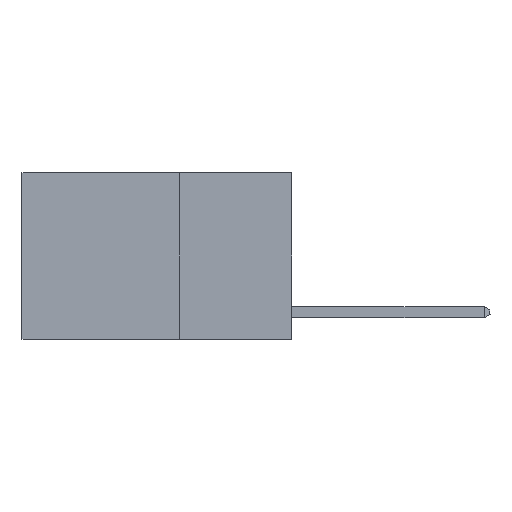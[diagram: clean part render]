
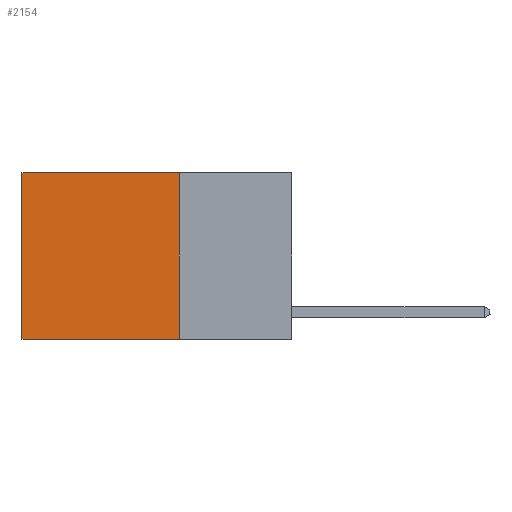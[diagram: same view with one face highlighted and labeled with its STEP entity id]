
A CAD part, left-side view. The second image highlights one B-rep face of the part: STEP entity #2154.
In plain terms, the highlighted planar face has unit normal (-1, 0, 0).
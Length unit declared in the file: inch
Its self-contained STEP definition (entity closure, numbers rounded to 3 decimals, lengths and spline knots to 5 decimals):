
#307 = LINE ( 'NONE', #6632, #8865 ) ;
#652 = EDGE_CURVE ( 'NONE', #10022, #9875, #307, .T. ) ;
#781 = LINE ( 'NONE', #2338, #8681 ) ;
#1498 = ORIENTED_EDGE ( 'NONE', *, *, #652, .T. ) ;
#1920 = DIRECTION ( 'NONE',  ( 0., 0., -1. ) ) ;
#2085 = AXIS2_PLACEMENT_3D ( 'NONE', #10280, #6936, #1920 ) ;
#2154 = ADVANCED_FACE ( 'NONE', ( #7402 ), #6077, .F. ) ;
#2165 = CARTESIAN_POINT ( 'NONE',  ( 0.2625, 0.6, 0. ) ) ;
#2338 = CARTESIAN_POINT ( 'NONE',  ( 0.2625, 0.25, 0. ) ) ;
#2395 = ORIENTED_EDGE ( 'NONE', *, *, #4912, .T. ) ;
#2463 = EDGE_CURVE ( 'NONE', #10022, #4652, #781, .T. ) ;
#3562 = LINE ( 'NONE', #7729, #7956 ) ;
#4652 = VERTEX_POINT ( 'NONE', #8123 ) ;
#4731 = CARTESIAN_POINT ( 'NONE',  ( 0.2625, 0.6, 0. ) ) ;
#4907 = VECTOR ( 'NONE', #8749, 39.37008 ) ;
#4912 = EDGE_CURVE ( 'NONE', #9875, #8847, #10698, .T. ) ;
#6077 = PLANE ( 'NONE',  #2085 ) ;
#6632 = CARTESIAN_POINT ( 'NONE',  ( 0.2625, 0.25, 0. ) ) ;
#6772 = EDGE_LOOP ( 'NONE', ( #2395, #9887, #7379, #1498 ) ) ;
#6936 = DIRECTION ( 'NONE',  ( 1., 0., 0. ) ) ;
#7379 = ORIENTED_EDGE ( 'NONE', *, *, #2463, .F. ) ;
#7402 = FACE_OUTER_BOUND ( 'NONE', #6772, .T. ) ;
#7729 = CARTESIAN_POINT ( 'NONE',  ( 0.2625, 0.25, -0.37 ) ) ;
#7862 = CARTESIAN_POINT ( 'NONE',  ( 0.2625, 0.25, 0. ) ) ;
#7956 = VECTOR ( 'NONE', #8550, 39.37008 ) ;
#8123 = CARTESIAN_POINT ( 'NONE',  ( 0.2625, 0.25, -0.37 ) ) ;
#8412 = EDGE_CURVE ( 'NONE', #4652, #8847, #3562, .T. ) ;
#8550 = DIRECTION ( 'NONE',  ( 0., 1., 0. ) ) ;
#8681 = VECTOR ( 'NONE', #9206, 39.37008 ) ;
#8749 = DIRECTION ( 'NONE',  ( 0., 0., -1. ) ) ;
#8847 = VERTEX_POINT ( 'NONE', #9685 ) ;
#8865 = VECTOR ( 'NONE', #9057, 39.37008 ) ;
#9057 = DIRECTION ( 'NONE',  ( 0., 1., 0. ) ) ;
#9206 = DIRECTION ( 'NONE',  ( 0., 0., -1. ) ) ;
#9685 = CARTESIAN_POINT ( 'NONE',  ( 0.2625, 0.6, -0.37 ) ) ;
#9875 = VERTEX_POINT ( 'NONE', #2165 ) ;
#9887 = ORIENTED_EDGE ( 'NONE', *, *, #8412, .F. ) ;
#10022 = VERTEX_POINT ( 'NONE', #7862 ) ;
#10280 = CARTESIAN_POINT ( 'NONE',  ( 0.2625, 0.25, 0. ) ) ;
#10698 = LINE ( 'NONE', #4731, #4907 ) ;
